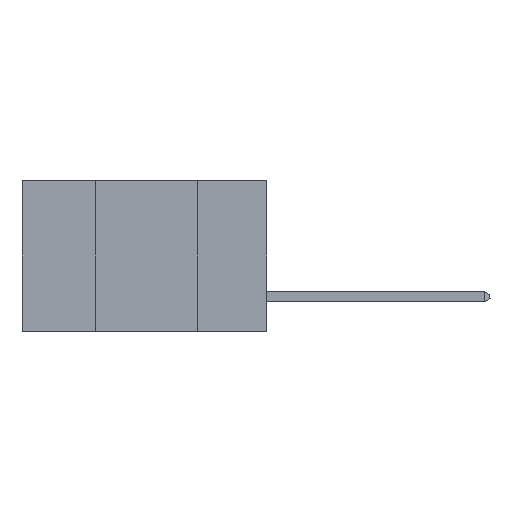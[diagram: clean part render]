
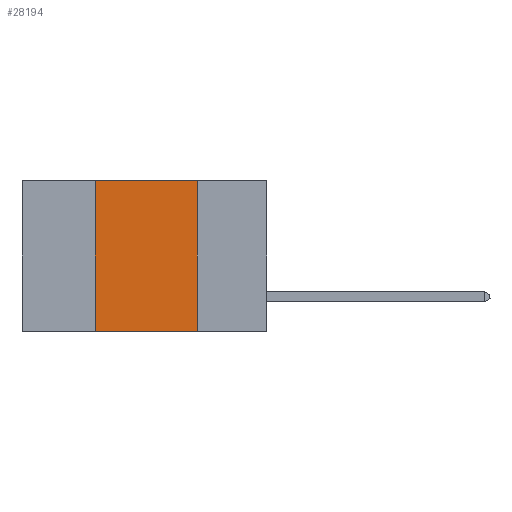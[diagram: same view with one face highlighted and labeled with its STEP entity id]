
A CAD part, left-side view. The second image highlights one B-rep face of the part: STEP entity #28194.
In plain terms, the highlighted planar face has unit normal (-1, 0, 0).
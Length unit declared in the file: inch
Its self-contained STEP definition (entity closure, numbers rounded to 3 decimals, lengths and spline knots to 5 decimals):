
#350 = CARTESIAN_POINT ( 'NONE',  ( 0., 0.17, -0.37 ) ) ;
#401 = VERTEX_POINT ( 'NONE', #28740 ) ;
#745 = DIRECTION ( 'NONE',  ( 0., -1., 0. ) ) ;
#920 = EDGE_CURVE ( 'NONE', #401, #1486, #15671, .T. ) ;
#1063 = DIRECTION ( 'NONE',  ( 0., 0., 1. ) ) ;
#1477 = PLANE ( 'NONE',  #24012 ) ;
#1486 = VERTEX_POINT ( 'NONE', #350 ) ;
#2096 = VECTOR ( 'NONE', #6646, 39.37008 ) ;
#2263 = DIRECTION ( 'NONE',  ( 0., 0., -1. ) ) ;
#2714 = VECTOR ( 'NONE', #745, 39.37008 ) ;
#3159 = CARTESIAN_POINT ( 'NONE',  ( 0., 0.42, 0. ) ) ;
#3521 = LINE ( 'NONE', #22504, #2096 ) ;
#3951 = DIRECTION ( 'NONE',  ( 0., 0., -1. ) ) ;
#5661 = EDGE_LOOP ( 'NONE', ( #16950, #10716, #22278, #11881 ) ) ;
#6400 = VECTOR ( 'NONE', #1063, 39.37008 ) ;
#6646 = DIRECTION ( 'NONE',  ( 0., -1., 0. ) ) ;
#8826 = VECTOR ( 'NONE', #2263, 39.37008 ) ;
#10716 = ORIENTED_EDGE ( 'NONE', *, *, #28716, .F. ) ;
#11031 = CARTESIAN_POINT ( 'NONE',  ( 0., 0.42, -0.37 ) ) ;
#11396 = FACE_OUTER_BOUND ( 'NONE', #5661, .T. ) ;
#11881 = ORIENTED_EDGE ( 'NONE', *, *, #27632, .T. ) ;
#13055 = EDGE_CURVE ( 'NONE', #23252, #16222, #16483, .T. ) ;
#13482 = LINE ( 'NONE', #16816, #2714 ) ;
#15404 = CARTESIAN_POINT ( 'NONE',  ( 0., 0.6, 0. ) ) ;
#15671 = LINE ( 'NONE', #27711, #8826 ) ;
#16222 = VERTEX_POINT ( 'NONE', #24078 ) ;
#16483 = LINE ( 'NONE', #3159, #6400 ) ;
#16816 = CARTESIAN_POINT ( 'NONE',  ( 0., 0.6, 0. ) ) ;
#16950 = ORIENTED_EDGE ( 'NONE', *, *, #920, .F. ) ;
#22278 = ORIENTED_EDGE ( 'NONE', *, *, #13055, .F. ) ;
#22504 = CARTESIAN_POINT ( 'NONE',  ( 0., 0.6, -0.37 ) ) ;
#23252 = VERTEX_POINT ( 'NONE', #11031 ) ;
#24012 = AXIS2_PLACEMENT_3D ( 'NONE', #15404, #24712, #3951 ) ;
#24078 = CARTESIAN_POINT ( 'NONE',  ( 0., 0.42, 0. ) ) ;
#24712 = DIRECTION ( 'NONE',  ( 1., 0., 0. ) ) ;
#27632 = EDGE_CURVE ( 'NONE', #23252, #1486, #3521, .T. ) ;
#27711 = CARTESIAN_POINT ( 'NONE',  ( 0., 0.17, 0. ) ) ;
#28194 = ADVANCED_FACE ( 'NONE', ( #11396 ), #1477, .F. ) ;
#28716 = EDGE_CURVE ( 'NONE', #16222, #401, #13482, .T. ) ;
#28740 = CARTESIAN_POINT ( 'NONE',  ( 0., 0.17, 0. ) ) ;
